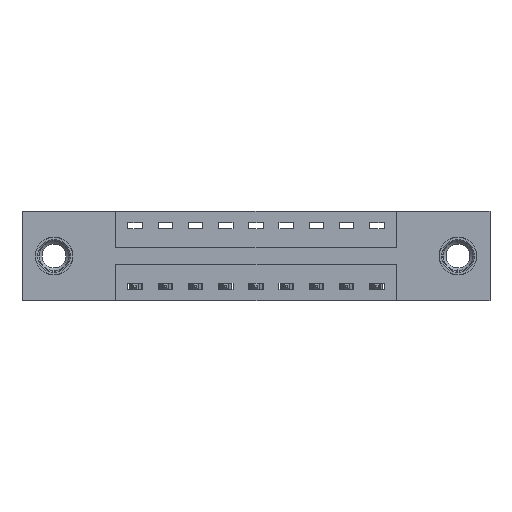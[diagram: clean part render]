
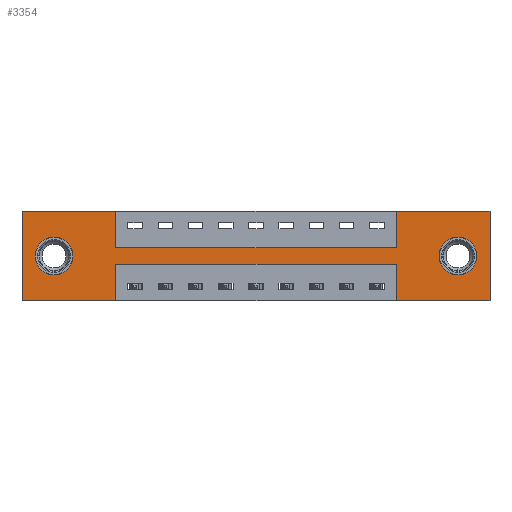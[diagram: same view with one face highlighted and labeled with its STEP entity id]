
A CAD part, front view. The second image highlights one B-rep face of the part: STEP entity #3354.
In plain terms, the highlighted planar face has unit normal (0, -1, 0).
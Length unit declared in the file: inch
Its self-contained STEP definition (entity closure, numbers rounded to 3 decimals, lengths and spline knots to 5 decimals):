
#121 = ORIENTED_EDGE ( 'NONE', *, *, #475, .T. ) ;
#155 = DIRECTION ( 'NONE',  ( 0., 0., 1. ) ) ;
#169 = DIRECTION ( 'NONE',  ( 0., 0., 1. ) ) ;
#214 = EDGE_CURVE ( 'NONE', #5841, #2335, #2174, .T. ) ;
#304 = VERTEX_POINT ( 'NONE', #6671 ) ;
#406 = CARTESIAN_POINT ( 'NONE',  ( 1.935, 0., 0. ) ) ;
#426 = EDGE_LOOP ( 'NONE', ( #5482, #591, #4379, #7528, #10792, #7021, #8929, #9810, #5940, #4177, #5523, #5819 ) ) ;
#459 = EDGE_CURVE ( 'NONE', #10511, #7649, #1913, .T. ) ;
#475 = EDGE_CURVE ( 'NONE', #5908, #9283, #7883, .T. ) ;
#522 = EDGE_CURVE ( 'NONE', #9283, #5908, #3519, .T. ) ;
#572 = PLANE ( 'NONE',  #9383 ) ;
#591 = ORIENTED_EDGE ( 'NONE', *, *, #1476, .F. ) ;
#792 = DIRECTION ( 'NONE',  ( -1., 0., 0. ) ) ;
#816 = DIRECTION ( 'NONE',  ( 1., 0., 0. ) ) ;
#959 = CARTESIAN_POINT ( 'NONE',  ( 0.3875, 0., -0.37 ) ) ;
#992 = CARTESIAN_POINT ( 'NONE',  ( 0.3875, 0., 0. ) ) ;
#1022 = CIRCLE ( 'NONE', #8820, 0.078 ) ;
#1071 = CARTESIAN_POINT ( 'NONE',  ( 0., 0., -0.37 ) ) ;
#1072 = DIRECTION ( 'NONE',  ( 0., 1., 0. ) ) ;
#1141 = CARTESIAN_POINT ( 'NONE',  ( 1.5475, 0., -0.37 ) ) ;
#1185 = DIRECTION ( 'NONE',  ( 1., 0., 0. ) ) ;
#1190 = DIRECTION ( 'NONE',  ( 0., 0., -1. ) ) ;
#1216 = DIRECTION ( 'NONE',  ( 0., 0., -1. ) ) ;
#1323 = CARTESIAN_POINT ( 'NONE',  ( 0.3875, 0., -0.22 ) ) ;
#1331 = LINE ( 'NONE', #6323, #3240 ) ;
#1351 = VERTEX_POINT ( 'NONE', #992 ) ;
#1395 = DIRECTION ( 'NONE',  ( 0., 0., 1. ) ) ;
#1476 = EDGE_CURVE ( 'NONE', #7649, #5469, #1331, .T. ) ;
#1488 = LINE ( 'NONE', #2951, #2286 ) ;
#1581 = CARTESIAN_POINT ( 'NONE',  ( 0., 0., -0.37 ) ) ;
#1589 = CARTESIAN_POINT ( 'NONE',  ( 0.1325, 0., -0.263 ) ) ;
#1651 = DIRECTION ( 'NONE',  ( 0., 0., -1. ) ) ;
#1801 = VECTOR ( 'NONE', #816, 39.37008 ) ;
#1873 = DIRECTION ( 'NONE',  ( 0., 1., 0. ) ) ;
#1913 = LINE ( 'NONE', #1141, #5139 ) ;
#2084 = CARTESIAN_POINT ( 'NONE',  ( 0., 0., -0.37 ) ) ;
#2152 = VECTOR ( 'NONE', #4653, 39.37008 ) ;
#2174 = LINE ( 'NONE', #2389, #4280 ) ;
#2286 = VECTOR ( 'NONE', #5678, 39.37008 ) ;
#2335 = VERTEX_POINT ( 'NONE', #8586 ) ;
#2389 = CARTESIAN_POINT ( 'NONE',  ( 0., 0., 0. ) ) ;
#2502 = DIRECTION ( 'NONE',  ( 0., 0., -1. ) ) ;
#2802 = EDGE_CURVE ( 'NONE', #1351, #4804, #10047, .T. ) ;
#2885 = AXIS2_PLACEMENT_3D ( 'NONE', #9705, #1873, #169 ) ;
#2915 = LINE ( 'NONE', #9904, #3275 ) ;
#2951 = CARTESIAN_POINT ( 'NONE',  ( 0.3875, 0., -0.37 ) ) ;
#3025 = VERTEX_POINT ( 'NONE', #7798 ) ;
#3031 = CARTESIAN_POINT ( 'NONE',  ( 1.5475, 0., -0.37 ) ) ;
#3065 = VECTOR ( 'NONE', #8068, 39.37008 ) ;
#3092 = CARTESIAN_POINT ( 'NONE',  ( 1.935, 0., 0. ) ) ;
#3129 = CARTESIAN_POINT ( 'NONE',  ( 0.3875, 0., 0. ) ) ;
#3240 = VECTOR ( 'NONE', #8958, 39.37008 ) ;
#3275 = VECTOR ( 'NONE', #1185, 39.37008 ) ;
#3284 = FACE_BOUND ( 'NONE', #6570, .T. ) ;
#3354 = ADVANCED_FACE ( 'NONE', ( #4875, #3284, #5840 ), #572, .T. ) ;
#3434 = EDGE_CURVE ( 'NONE', #3025, #6968, #1022, .T. ) ;
#3506 = VERTEX_POINT ( 'NONE', #10363 ) ;
#3519 = CIRCLE ( 'NONE', #9356, 0.078 ) ;
#3653 = VECTOR ( 'NONE', #792, 39.37008 ) ;
#4089 = DIRECTION ( 'NONE',  ( 0., -1., 0. ) ) ;
#4177 = ORIENTED_EDGE ( 'NONE', *, *, #9349, .F. ) ;
#4224 = CARTESIAN_POINT ( 'NONE',  ( 1.8025, 0., -0.263 ) ) ;
#4252 = CARTESIAN_POINT ( 'NONE',  ( 1.8025, 0., -0.107 ) ) ;
#4280 = VECTOR ( 'NONE', #1395, 39.37008 ) ;
#4379 = ORIENTED_EDGE ( 'NONE', *, *, #459, .F. ) ;
#4449 = LINE ( 'NONE', #10556, #1801 ) ;
#4551 = EDGE_CURVE ( 'NONE', #7236, #304, #10912, .T. ) ;
#4612 = CARTESIAN_POINT ( 'NONE',  ( 1.5475, 0., 0. ) ) ;
#4653 = DIRECTION ( 'NONE',  ( 1., 0., 0. ) ) ;
#4804 = VERTEX_POINT ( 'NONE', #8784 ) ;
#4875 = FACE_BOUND ( 'NONE', #6682, .T. ) ;
#5089 = LINE ( 'NONE', #8579, #3653 ) ;
#5139 = VECTOR ( 'NONE', #6295, 39.37008 ) ;
#5269 = VERTEX_POINT ( 'NONE', #4612 ) ;
#5317 = LINE ( 'NONE', #1071, #3065 ) ;
#5331 = DIRECTION ( 'NONE',  ( 0., 0., 1. ) ) ;
#5386 = EDGE_CURVE ( 'NONE', #5469, #10173, #1488, .T. ) ;
#5392 = CARTESIAN_POINT ( 'NONE',  ( 0.3875, 0., -0.15 ) ) ;
#5469 = VERTEX_POINT ( 'NONE', #1323 ) ;
#5482 = ORIENTED_EDGE ( 'NONE', *, *, #5386, .F. ) ;
#5493 = CARTESIAN_POINT ( 'NONE',  ( 1.8025, 0., -0.185 ) ) ;
#5523 = ORIENTED_EDGE ( 'NONE', *, *, #214, .F. ) ;
#5678 = DIRECTION ( 'NONE',  ( 0., 0., -1. ) ) ;
#5819 = ORIENTED_EDGE ( 'NONE', *, *, #7548, .F. ) ;
#5840 = FACE_OUTER_BOUND ( 'NONE', #426, .T. ) ;
#5841 = VERTEX_POINT ( 'NONE', #2084 ) ;
#5908 = VERTEX_POINT ( 'NONE', #4252 ) ;
#5940 = ORIENTED_EDGE ( 'NONE', *, *, #2802, .F. ) ;
#5972 = CIRCLE ( 'NONE', #2885, 0.078 ) ;
#6295 = DIRECTION ( 'NONE',  ( 0., 0., 1. ) ) ;
#6323 = CARTESIAN_POINT ( 'NONE',  ( 0.3875, 0., -0.22 ) ) ;
#6383 = VECTOR ( 'NONE', #5331, 39.37008 ) ;
#6459 = CARTESIAN_POINT ( 'NONE',  ( 1.5475, 0., -0.22 ) ) ;
#6570 = EDGE_LOOP ( 'NONE', ( #7235, #6964 ) ) ;
#6671 = CARTESIAN_POINT ( 'NONE',  ( 1.935, 0., -0.37 ) ) ;
#6682 = EDGE_LOOP ( 'NONE', ( #121, #9758 ) ) ;
#6964 = ORIENTED_EDGE ( 'NONE', *, *, #7127, .T. ) ;
#6968 = VERTEX_POINT ( 'NONE', #1589 ) ;
#7021 = ORIENTED_EDGE ( 'NONE', *, *, #8708, .F. ) ;
#7058 = EDGE_CURVE ( 'NONE', #4804, #3506, #10607, .T. ) ;
#7127 = EDGE_CURVE ( 'NONE', #6968, #3025, #5972, .T. ) ;
#7235 = ORIENTED_EDGE ( 'NONE', *, *, #3434, .T. ) ;
#7236 = VERTEX_POINT ( 'NONE', #406 ) ;
#7528 = ORIENTED_EDGE ( 'NONE', *, *, #10269, .F. ) ;
#7548 = EDGE_CURVE ( 'NONE', #10173, #5841, #5317, .T. ) ;
#7649 = VERTEX_POINT ( 'NONE', #6459 ) ;
#7798 = CARTESIAN_POINT ( 'NONE',  ( 0.1325, 0., -0.107 ) ) ;
#7843 = DIRECTION ( 'NONE',  ( 0., 1., 0. ) ) ;
#7883 = CIRCLE ( 'NONE', #9346, 0.078 ) ;
#8012 = CARTESIAN_POINT ( 'NONE',  ( 1.8025, 0., -0.185 ) ) ;
#8068 = DIRECTION ( 'NONE',  ( -1., 0., 0. ) ) ;
#8421 = CARTESIAN_POINT ( 'NONE',  ( 0.1325, 0., -0.185 ) ) ;
#8579 = CARTESIAN_POINT ( 'NONE',  ( 0., 0., -0.37 ) ) ;
#8586 = CARTESIAN_POINT ( 'NONE',  ( 0., 0., 0. ) ) ;
#8708 = EDGE_CURVE ( 'NONE', #5269, #7236, #2915, .T. ) ;
#8784 = CARTESIAN_POINT ( 'NONE',  ( 0.3875, 0., -0.15 ) ) ;
#8820 = AXIS2_PLACEMENT_3D ( 'NONE', #8421, #7843, #155 ) ;
#8929 = ORIENTED_EDGE ( 'NONE', *, *, #11139, .F. ) ;
#8958 = DIRECTION ( 'NONE',  ( -1., 0., 0. ) ) ;
#9283 = VERTEX_POINT ( 'NONE', #4224 ) ;
#9346 = AXIS2_PLACEMENT_3D ( 'NONE', #5493, #9461, #1651 ) ;
#9349 = EDGE_CURVE ( 'NONE', #2335, #1351, #4449, .T. ) ;
#9356 = AXIS2_PLACEMENT_3D ( 'NONE', #8012, #1072, #1190 ) ;
#9383 = AXIS2_PLACEMENT_3D ( 'NONE', #1581, #4089, #10988 ) ;
#9461 = DIRECTION ( 'NONE',  ( 0., 1., 0. ) ) ;
#9631 = CARTESIAN_POINT ( 'NONE',  ( 1.5475, 0., 0. ) ) ;
#9705 = CARTESIAN_POINT ( 'NONE',  ( 0.1325, 0., -0.185 ) ) ;
#9758 = ORIENTED_EDGE ( 'NONE', *, *, #522, .T. ) ;
#9810 = ORIENTED_EDGE ( 'NONE', *, *, #7058, .F. ) ;
#9904 = CARTESIAN_POINT ( 'NONE',  ( 0., 0., 0. ) ) ;
#10047 = LINE ( 'NONE', #3129, #10748 ) ;
#10131 = VECTOR ( 'NONE', #2502, 39.37008 ) ;
#10173 = VERTEX_POINT ( 'NONE', #959 ) ;
#10269 = EDGE_CURVE ( 'NONE', #304, #10511, #5089, .T. ) ;
#10363 = CARTESIAN_POINT ( 'NONE',  ( 1.5475, 0., -0.15 ) ) ;
#10511 = VERTEX_POINT ( 'NONE', #3031 ) ;
#10556 = CARTESIAN_POINT ( 'NONE',  ( 0., 0., 0. ) ) ;
#10605 = LINE ( 'NONE', #9631, #6383 ) ;
#10607 = LINE ( 'NONE', #5392, #2152 ) ;
#10748 = VECTOR ( 'NONE', #1216, 39.37008 ) ;
#10792 = ORIENTED_EDGE ( 'NONE', *, *, #4551, .F. ) ;
#10912 = LINE ( 'NONE', #3092, #10131 ) ;
#10988 = DIRECTION ( 'NONE',  ( 0., 0., -1. ) ) ;
#11139 = EDGE_CURVE ( 'NONE', #3506, #5269, #10605, .T. ) ;
